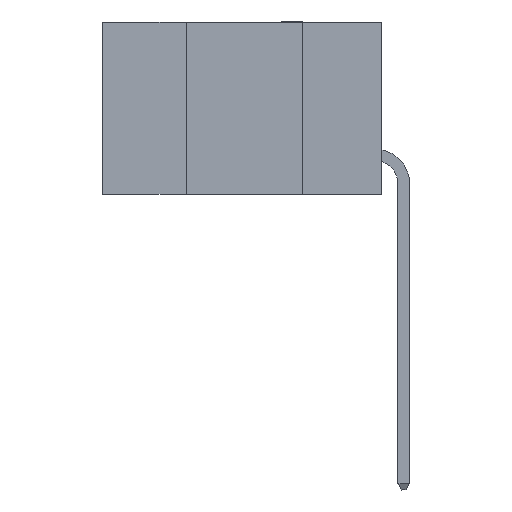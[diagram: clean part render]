
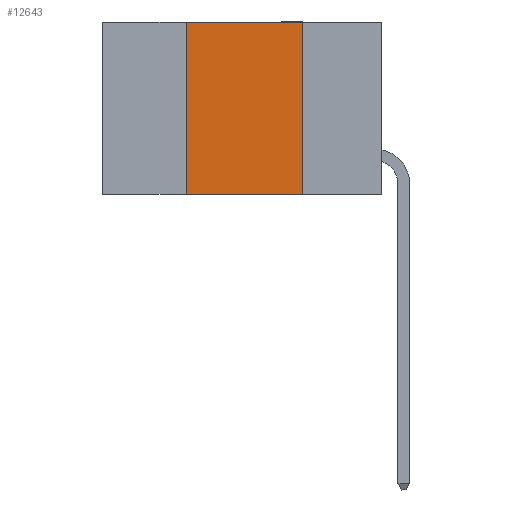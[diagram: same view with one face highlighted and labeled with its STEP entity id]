
A CAD part, left-side view. The second image highlights one B-rep face of the part: STEP entity #12643.
In plain terms, the highlighted planar face has unit normal (-1, 0, 0).
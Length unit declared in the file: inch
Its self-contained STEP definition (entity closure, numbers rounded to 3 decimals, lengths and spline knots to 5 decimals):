
#141 = CARTESIAN_POINT ( 'NONE',  ( 0., 0.42, -0.37 ) ) ;
#628 = VERTEX_POINT ( 'NONE', #16366 ) ;
#694 = AXIS2_PLACEMENT_3D ( 'NONE', #10869, #14937, #6853 ) ;
#812 = LINE ( 'NONE', #10020, #14833 ) ;
#1675 = VERTEX_POINT ( 'NONE', #141 ) ;
#2646 = VECTOR ( 'NONE', #15151, 39.37008 ) ;
#3394 = CARTESIAN_POINT ( 'NONE',  ( 0., 0.17, 0. ) ) ;
#3913 = LINE ( 'NONE', #3394, #10662 ) ;
#4375 = CARTESIAN_POINT ( 'NONE',  ( 0., 0.6, -0.37 ) ) ;
#5374 = EDGE_LOOP ( 'NONE', ( #7365, #5902, #9065, #11399 ) ) ;
#5518 = PLANE ( 'NONE',  #694 ) ;
#5902 = ORIENTED_EDGE ( 'NONE', *, *, #8039, .F. ) ;
#5917 = DIRECTION ( 'NONE',  ( 0., -1., 0. ) ) ;
#6281 = VERTEX_POINT ( 'NONE', #10502 ) ;
#6357 = CARTESIAN_POINT ( 'NONE',  ( 0., 0.17, -0.37 ) ) ;
#6853 = DIRECTION ( 'NONE',  ( 0., 0., -1. ) ) ;
#7302 = DIRECTION ( 'NONE',  ( 0., 0., 1. ) ) ;
#7365 = ORIENTED_EDGE ( 'NONE', *, *, #16706, .F. ) ;
#8039 = EDGE_CURVE ( 'NONE', #628, #6281, #11567, .T. ) ;
#8571 = EDGE_CURVE ( 'NONE', #1675, #8817, #9424, .T. ) ;
#8817 = VERTEX_POINT ( 'NONE', #6357 ) ;
#9065 = ORIENTED_EDGE ( 'NONE', *, *, #10418, .F. ) ;
#9424 = LINE ( 'NONE', #4375, #2646 ) ;
#10020 = CARTESIAN_POINT ( 'NONE',  ( 0., 0.42, 0. ) ) ;
#10418 = EDGE_CURVE ( 'NONE', #1675, #628, #812, .T. ) ;
#10502 = CARTESIAN_POINT ( 'NONE',  ( 0., 0.17, 0. ) ) ;
#10662 = VECTOR ( 'NONE', #14194, 39.37008 ) ;
#10869 = CARTESIAN_POINT ( 'NONE',  ( 0., 0.6, 0. ) ) ;
#11131 = VECTOR ( 'NONE', #5917, 39.37008 ) ;
#11399 = ORIENTED_EDGE ( 'NONE', *, *, #8571, .T. ) ;
#11567 = LINE ( 'NONE', #16674, #11131 ) ;
#12643 = ADVANCED_FACE ( 'NONE', ( #16284 ), #5518, .F. ) ;
#14194 = DIRECTION ( 'NONE',  ( 0., 0., -1. ) ) ;
#14833 = VECTOR ( 'NONE', #7302, 39.37008 ) ;
#14937 = DIRECTION ( 'NONE',  ( 1., 0., 0. ) ) ;
#15151 = DIRECTION ( 'NONE',  ( 0., -1., 0. ) ) ;
#16284 = FACE_OUTER_BOUND ( 'NONE', #5374, .T. ) ;
#16366 = CARTESIAN_POINT ( 'NONE',  ( 0., 0.42, 0. ) ) ;
#16674 = CARTESIAN_POINT ( 'NONE',  ( 0., 0.6, 0. ) ) ;
#16706 = EDGE_CURVE ( 'NONE', #6281, #8817, #3913, .T. ) ;
